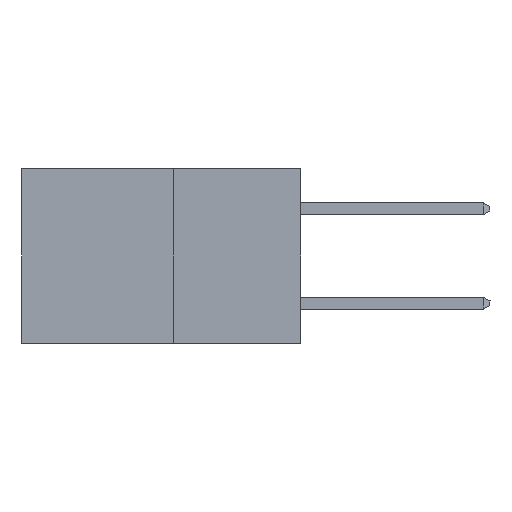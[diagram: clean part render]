
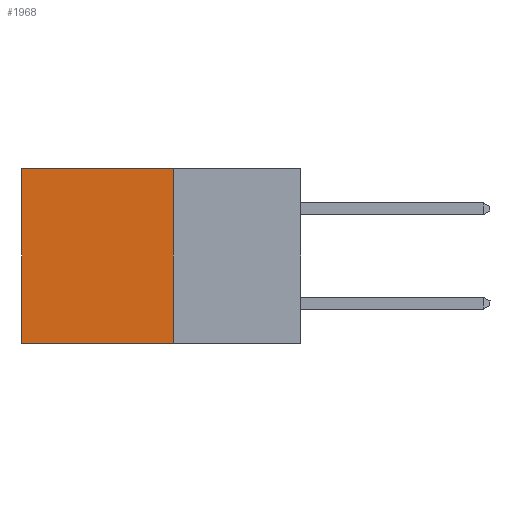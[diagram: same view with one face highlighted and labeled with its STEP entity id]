
A CAD part, left-side view. The second image highlights one B-rep face of the part: STEP entity #1968.
In plain terms, the highlighted planar face has unit normal (-1, 0, 0).
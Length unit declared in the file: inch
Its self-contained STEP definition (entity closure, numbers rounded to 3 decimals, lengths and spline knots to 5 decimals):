
#81 = VERTEX_POINT ( 'NONE', #2562 ) ;
#306 = VECTOR ( 'NONE', #2660, 39.37008 ) ;
#501 = ORIENTED_EDGE ( 'NONE', *, *, #740, .T. ) ;
#643 = CARTESIAN_POINT ( 'NONE',  ( 0.277, 0.59, -0.37 ) ) ;
#677 = VECTOR ( 'NONE', #12513, 39.37008 ) ;
#740 = EDGE_CURVE ( 'NONE', #81, #9804, #1414, .T. ) ;
#983 = ORIENTED_EDGE ( 'NONE', *, *, #10638, .T. ) ;
#1414 = LINE ( 'NONE', #10749, #12028 ) ;
#1861 = CARTESIAN_POINT ( 'NONE',  ( 0.277, 0.27, -0.37 ) ) ;
#1968 = ADVANCED_FACE ( 'NONE', ( #7526 ), #11629, .F. ) ;
#2296 = ORIENTED_EDGE ( 'NONE', *, *, #12018, .F. ) ;
#2562 = CARTESIAN_POINT ( 'NONE',  ( 0.277, 0.27, 0. ) ) ;
#2660 = DIRECTION ( 'NONE',  ( 0., 0., -1. ) ) ;
#3065 = EDGE_CURVE ( 'NONE', #12997, #11505, #5588, .T. ) ;
#3146 = DIRECTION ( 'NONE',  ( 0., 1., 0. ) ) ;
#3653 = CARTESIAN_POINT ( 'NONE',  ( 0.277, 0.59, 0. ) ) ;
#4106 = ORIENTED_EDGE ( 'NONE', *, *, #3065, .F. ) ;
#4521 = EDGE_LOOP ( 'NONE', ( #983, #4106, #2296, #501 ) ) ;
#4617 = VECTOR ( 'NONE', #4860, 39.37008 ) ;
#4860 = DIRECTION ( 'NONE',  ( 0., 0., -1. ) ) ;
#4946 = LINE ( 'NONE', #643, #4617 ) ;
#4953 = CARTESIAN_POINT ( 'NONE',  ( 0.277, 0.27, -0.37 ) ) ;
#5588 = LINE ( 'NONE', #11164, #677 ) ;
#7016 = CARTESIAN_POINT ( 'NONE',  ( 0.277, 0.59, -0.37 ) ) ;
#7526 = FACE_OUTER_BOUND ( 'NONE', #4521, .T. ) ;
#7781 = CARTESIAN_POINT ( 'NONE',  ( 0.277, 0.27, -0.37 ) ) ;
#8279 = LINE ( 'NONE', #7781, #306 ) ;
#9804 = VERTEX_POINT ( 'NONE', #3653 ) ;
#10638 = EDGE_CURVE ( 'NONE', #9804, #11505, #4946, .T. ) ;
#10749 = CARTESIAN_POINT ( 'NONE',  ( 0.277, 0.27, 0. ) ) ;
#11164 = CARTESIAN_POINT ( 'NONE',  ( 0.277, 0.27, -0.37 ) ) ;
#11505 = VERTEX_POINT ( 'NONE', #7016 ) ;
#11629 = PLANE ( 'NONE',  #11737 ) ;
#11737 = AXIS2_PLACEMENT_3D ( 'NONE', #1861, #12536, #12515 ) ;
#12018 = EDGE_CURVE ( 'NONE', #81, #12997, #8279, .T. ) ;
#12028 = VECTOR ( 'NONE', #3146, 39.37008 ) ;
#12513 = DIRECTION ( 'NONE',  ( 0., 1., 0. ) ) ;
#12515 = DIRECTION ( 'NONE',  ( 0., 0., -1. ) ) ;
#12536 = DIRECTION ( 'NONE',  ( 1., 0., 0. ) ) ;
#12997 = VERTEX_POINT ( 'NONE', #4953 ) ;
